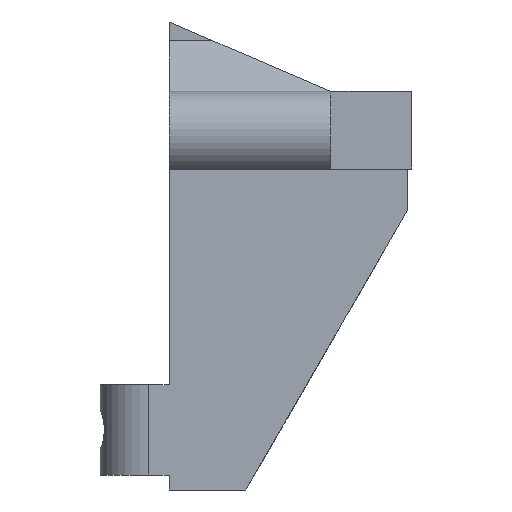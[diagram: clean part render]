
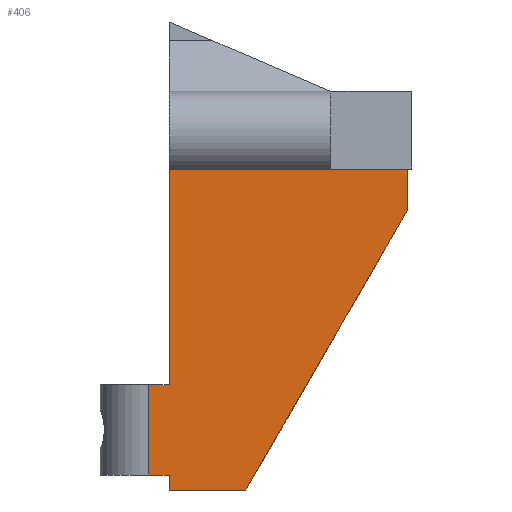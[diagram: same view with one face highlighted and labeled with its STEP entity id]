
A CAD part, left-side view. The second image highlights one B-rep face of the part: STEP entity #406.
In plain terms, the highlighted planar face has unit normal (-1, 0, 0).
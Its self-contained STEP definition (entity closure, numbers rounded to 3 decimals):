
#7 = ORIENTED_EDGE ( 'NONE', *, *, #40, .F. ) ;
#28 = ORIENTED_EDGE ( 'NONE', *, *, #830, .F. ) ;
#29 = LINE ( 'NONE', #468, #165 ) ;
#40 = EDGE_CURVE ( 'NONE', #684, #1180, #1100, .T. ) ;
#43 = DIRECTION ( 'NONE',  ( 0., 1., 0. ) ) ;
#44 = VECTOR ( 'NONE', #258, 1000. ) ;
#65 = EDGE_CURVE ( 'NONE', #682, #945, #1068, .T. ) ;
#66 = DIRECTION ( 'NONE',  ( 0., 0., 1. ) ) ;
#71 = VECTOR ( 'NONE', #397, 1000. ) ;
#85 = CARTESIAN_POINT ( 'NONE',  ( -4.8, -8.6, -57.74 ) ) ;
#98 = DIRECTION ( 'NONE',  ( 0., -1., 0. ) ) ;
#105 = LINE ( 'NONE', #856, #44 ) ;
#123 = CARTESIAN_POINT ( 'NONE',  ( -4.8, 6.946, -56.257 ) ) ;
#132 = VERTEX_POINT ( 'NONE', #704 ) ;
#140 = CARTESIAN_POINT ( 'NONE',  ( -4.8, -24.622, -29.989 ) ) ;
#146 = CARTESIAN_POINT ( 'NONE',  ( -4.8, -1., -57.74 ) ) ;
#159 = PLANE ( 'NONE',  #461 ) ;
#165 = VECTOR ( 'NONE', #478, 1000. ) ;
#193 = ORIENTED_EDGE ( 'NONE', *, *, #300, .F. ) ;
#215 = EDGE_CURVE ( 'NONE', #945, #723, #377, .T. ) ;
#254 = CARTESIAN_POINT ( 'NONE',  ( -4.8, 1., -56.257 ) ) ;
#258 = DIRECTION ( 'NONE',  ( 0., 0., -1. ) ) ;
#262 = CARTESIAN_POINT ( 'NONE',  ( -4.8, -1., -56.257 ) ) ;
#263 = EDGE_CURVE ( 'NONE', #657, #684, #290, .T. ) ;
#290 = LINE ( 'NONE', #146, #742 ) ;
#294 = CARTESIAN_POINT ( 'NONE',  ( -4.8, 6.946, -47.307 ) ) ;
#300 = EDGE_CURVE ( 'NONE', #132, #1101, #105, .T. ) ;
#306 = DIRECTION ( 'NONE',  ( 0., 1., 0. ) ) ;
#308 = ORIENTED_EDGE ( 'NONE', *, *, #314, .F. ) ;
#314 = EDGE_CURVE ( 'NONE', #1101, #657, #29, .T. ) ;
#357 = ORIENTED_EDGE ( 'NONE', *, *, #906, .F. ) ;
#374 = CARTESIAN_POINT ( 'NONE',  ( -4.8, 0., 0. ) ) ;
#377 = LINE ( 'NONE', #1104, #1151 ) ;
#397 = DIRECTION ( 'NONE',  ( 0., 0., 1. ) ) ;
#406 = ADVANCED_FACE ( 'NONE', ( #1222 ), #159, .T. ) ;
#410 = CARTESIAN_POINT ( 'NONE',  ( -4.8, 1., -47.307 ) ) ;
#442 = CARTESIAN_POINT ( 'NONE',  ( -4.8, -1., -47.307 ) ) ;
#446 = DIRECTION ( 'NONE',  ( 0., -1., 0. ) ) ;
#461 = AXIS2_PLACEMENT_3D ( 'NONE', #374, #565, #66 ) ;
#468 = CARTESIAN_POINT ( 'NONE',  ( -4.8, -8.6, -57.74 ) ) ;
#472 = VECTOR ( 'NONE', #98, 1000. ) ;
#478 = DIRECTION ( 'NONE',  ( 0., 0.5, -0.866 ) ) ;
#490 = LINE ( 'NONE', #1186, #638 ) ;
#509 = CARTESIAN_POINT ( 'NONE',  ( -4.8, -1., -25.99 ) ) ;
#565 = DIRECTION ( 'NONE',  ( -1., 0., 0. ) ) ;
#572 = ORIENTED_EDGE ( 'NONE', *, *, #65, .F. ) ;
#638 = VECTOR ( 'NONE', #446, 1000. ) ;
#650 = CARTESIAN_POINT ( 'NONE',  ( -4.8, 1., -44.757 ) ) ;
#657 = VERTEX_POINT ( 'NONE', #85 ) ;
#682 = VERTEX_POINT ( 'NONE', #410 ) ;
#684 = VERTEX_POINT ( 'NONE', #960 ) ;
#704 = CARTESIAN_POINT ( 'NONE',  ( -4.8, -24.622, -25.99 ) ) ;
#707 = LINE ( 'NONE', #650, #931 ) ;
#723 = VERTEX_POINT ( 'NONE', #509 ) ;
#742 = VECTOR ( 'NONE', #43, 1000. ) ;
#756 = ORIENTED_EDGE ( 'NONE', *, *, #215, .F. ) ;
#767 = CARTESIAN_POINT ( 'NONE',  ( -4.8, -1., -25.99 ) ) ;
#830 = EDGE_CURVE ( 'NONE', #1180, #1122, #860, .T. ) ;
#836 = DIRECTION ( 'NONE',  ( 0., 0., 1. ) ) ;
#856 = CARTESIAN_POINT ( 'NONE',  ( -4.8, -24.622, -29.989 ) ) ;
#860 = LINE ( 'NONE', #123, #1187 ) ;
#906 = EDGE_CURVE ( 'NONE', #723, #132, #490, .T. ) ;
#907 = ORIENTED_EDGE ( 'NONE', *, *, #263, .F. ) ;
#931 = VECTOR ( 'NONE', #1205, 1000. ) ;
#945 = VERTEX_POINT ( 'NONE', #442 ) ;
#960 = CARTESIAN_POINT ( 'NONE',  ( -4.8, -1., -57.74 ) ) ;
#974 = EDGE_CURVE ( 'NONE', #682, #1122, #707, .T. ) ;
#979 = EDGE_LOOP ( 'NONE', ( #1024, #28, #7, #907, #308, #193, #357, #756, #572 ) ) ;
#1024 = ORIENTED_EDGE ( 'NONE', *, *, #974, .T. ) ;
#1068 = LINE ( 'NONE', #294, #472 ) ;
#1100 = LINE ( 'NONE', #767, #71 ) ;
#1101 = VERTEX_POINT ( 'NONE', #140 ) ;
#1104 = CARTESIAN_POINT ( 'NONE',  ( -4.8, -1., -25.99 ) ) ;
#1122 = VERTEX_POINT ( 'NONE', #254 ) ;
#1151 = VECTOR ( 'NONE', #836, 1000. ) ;
#1180 = VERTEX_POINT ( 'NONE', #262 ) ;
#1186 = CARTESIAN_POINT ( 'NONE',  ( -4.8, -24.622, -25.99 ) ) ;
#1187 = VECTOR ( 'NONE', #306, 1000. ) ;
#1205 = DIRECTION ( 'NONE',  ( 0., 0., -1. ) ) ;
#1222 = FACE_OUTER_BOUND ( 'NONE', #979, .T. ) ;
